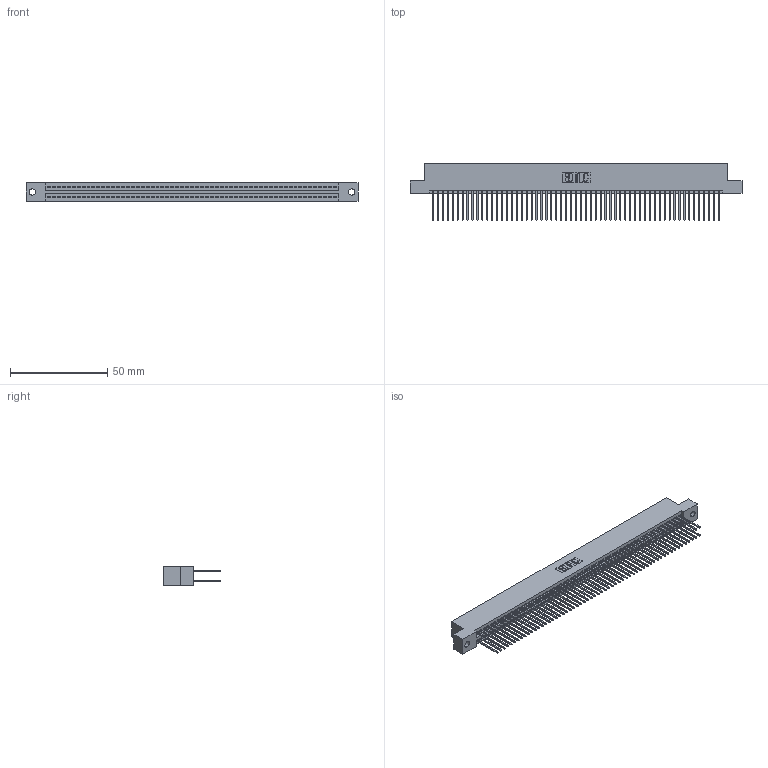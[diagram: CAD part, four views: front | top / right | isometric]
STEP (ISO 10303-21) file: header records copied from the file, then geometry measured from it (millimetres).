
FILE_DESCRIPTION (( 'STEP AP203' ), '1' );
FILE_NAME ('395-118-540-202.STEP', '2018-12-02T06:43:55', ( '' ), ( '' ), 'SwSTEP 2.0', 'SolidWorks 2016', '' );
FILE_SCHEMA (( 'CONFIG_CONTROL_DESIGN' ));
Length unit declared in the file: inch
Products named in the file (3): 345-292-001_345-293-140; 395-118-540-202; 345 Part_Flush Mounting Lugs - 0.128 Dia
Assembly tree (119 placements, depth 2):
  395-118-540-202
    345 Part_Flush Mounting Lugs - 0.128 Dia
    345-292-001_345-293-140  x118
Bounding box: 171.07 x 29.13 x 9.4 mm (x, y, z)
Volume: 17186.3 mm3; surface area: 27536.1 mm2
Topology: 119 solids, 119 shells, 6026 faces, 17923 edges, 11790 vertices
Faces by surface type: plane 3974, cylinder 2052
Entity records: 44025 total; most frequent: CARTESIAN_POINT 7364, ORIENTED_EDGE 7298, DIRECTION 6473, EDGE_CURVE 3649, VECTOR 3281, LINE 3281, VERTEX_POINT 2430, AXIS2_PLACEMENT_3D 1596
